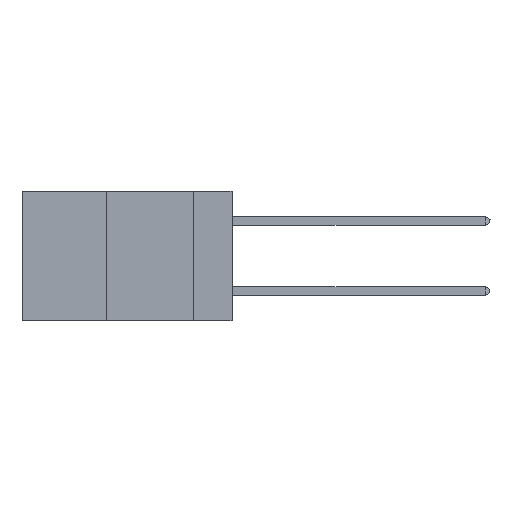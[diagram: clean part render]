
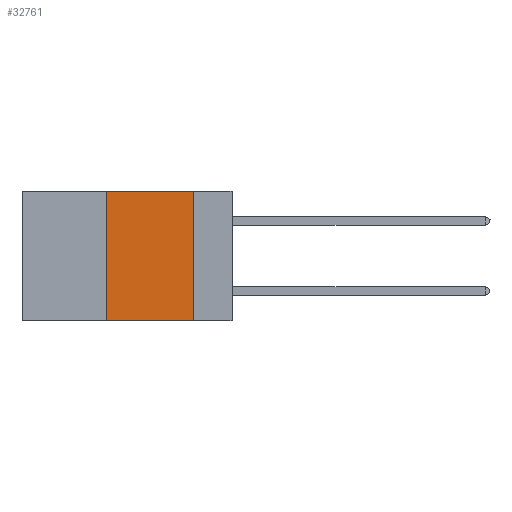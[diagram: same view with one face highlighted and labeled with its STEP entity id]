
A CAD part, left-side view. The second image highlights one B-rep face of the part: STEP entity #32761.
In plain terms, the highlighted planar face has unit normal (-1, 0, 0).
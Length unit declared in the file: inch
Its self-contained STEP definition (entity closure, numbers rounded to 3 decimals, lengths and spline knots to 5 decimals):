
#1113 = LINE ( 'NONE', #8393, #29838 ) ;
#1532 = ORIENTED_EDGE ( 'NONE', *, *, #41612, .F. ) ;
#4795 = LINE ( 'NONE', #13061, #47682 ) ;
#5856 = VERTEX_POINT ( 'NONE', #20326 ) ;
#8296 = DIRECTION ( 'NONE',  ( 0., 0., -1. ) ) ;
#8393 = CARTESIAN_POINT ( 'NONE',  ( 0., 0.36, 0. ) ) ;
#10670 = CARTESIAN_POINT ( 'NONE',  ( 0., 0.11, -0.37 ) ) ;
#11053 = CARTESIAN_POINT ( 'NONE',  ( 0., 0.11, 0. ) ) ;
#11529 = EDGE_CURVE ( 'NONE', #31787, #44706, #45987, .T. ) ;
#12065 = CARTESIAN_POINT ( 'NONE',  ( 0., 0.11, 0. ) ) ;
#13061 = CARTESIAN_POINT ( 'NONE',  ( 0., 0.6, 0. ) ) ;
#14211 = CARTESIAN_POINT ( 'NONE',  ( 0., 0.6, 0. ) ) ;
#17839 = EDGE_CURVE ( 'NONE', #5856, #44706, #18574, .T. ) ;
#17981 = PLANE ( 'NONE',  #30429 ) ;
#18574 = LINE ( 'NONE', #33906, #21494 ) ;
#20326 = CARTESIAN_POINT ( 'NONE',  ( 0., 0.36, -0.37 ) ) ;
#21494 = VECTOR ( 'NONE', #45703, 39.37008 ) ;
#21837 = VERTEX_POINT ( 'NONE', #46659 ) ;
#25792 = FACE_OUTER_BOUND ( 'NONE', #35993, .T. ) ;
#26607 = ORIENTED_EDGE ( 'NONE', *, *, #26785, .F. ) ;
#26785 = EDGE_CURVE ( 'NONE', #21837, #31787, #4795, .T. ) ;
#29838 = VECTOR ( 'NONE', #31271, 39.37008 ) ;
#30292 = DIRECTION ( 'NONE',  ( 1., 0., 0. ) ) ;
#30429 = AXIS2_PLACEMENT_3D ( 'NONE', #14211, #30292, #33314 ) ;
#31271 = DIRECTION ( 'NONE',  ( 0., 0., 1. ) ) ;
#31787 = VERTEX_POINT ( 'NONE', #11053 ) ;
#32414 = DIRECTION ( 'NONE',  ( 0., -1., 0. ) ) ;
#32761 = ADVANCED_FACE ( 'NONE', ( #25792 ), #17981, .F. ) ;
#33314 = DIRECTION ( 'NONE',  ( 0., 0., -1. ) ) ;
#33906 = CARTESIAN_POINT ( 'NONE',  ( 0., 0.6, -0.37 ) ) ;
#35993 = EDGE_LOOP ( 'NONE', ( #40480, #26607, #1532, #48392 ) ) ;
#40455 = VECTOR ( 'NONE', #8296, 39.37008 ) ;
#40480 = ORIENTED_EDGE ( 'NONE', *, *, #11529, .F. ) ;
#41612 = EDGE_CURVE ( 'NONE', #5856, #21837, #1113, .T. ) ;
#44706 = VERTEX_POINT ( 'NONE', #10670 ) ;
#45703 = DIRECTION ( 'NONE',  ( 0., -1., 0. ) ) ;
#45987 = LINE ( 'NONE', #12065, #40455 ) ;
#46659 = CARTESIAN_POINT ( 'NONE',  ( 0., 0.36, 0. ) ) ;
#47682 = VECTOR ( 'NONE', #32414, 39.37008 ) ;
#48392 = ORIENTED_EDGE ( 'NONE', *, *, #17839, .T. ) ;
